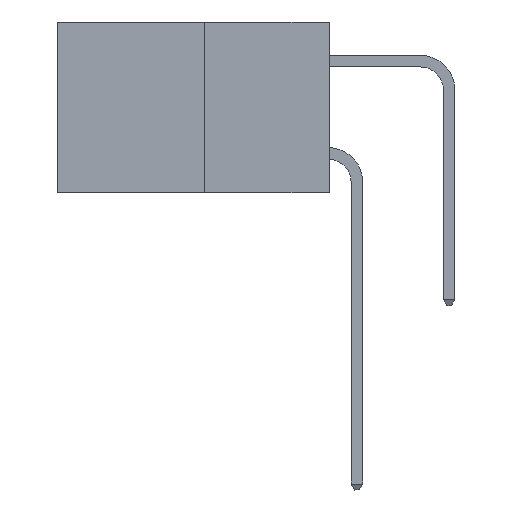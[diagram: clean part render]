
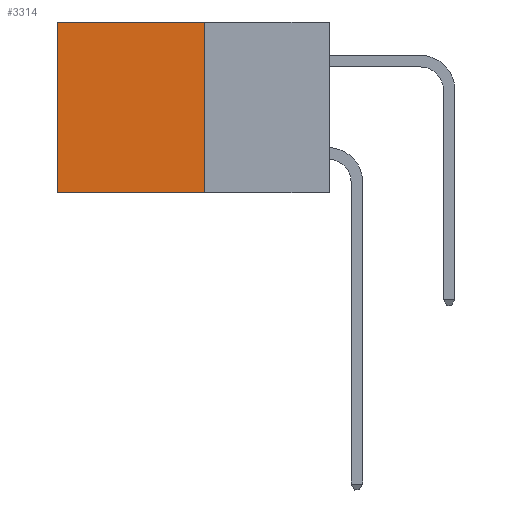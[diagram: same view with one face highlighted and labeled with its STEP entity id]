
A CAD part, left-side view. The second image highlights one B-rep face of the part: STEP entity #3314.
In plain terms, the highlighted planar face has unit normal (-1, 0, 0).
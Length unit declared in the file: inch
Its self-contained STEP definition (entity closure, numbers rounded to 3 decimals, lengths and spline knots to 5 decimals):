
#16 = AXIS2_PLACEMENT_3D ( 'NONE', #9712, #11095, #9691 ) ;
#469 = VECTOR ( 'NONE', #6134, 39.37008 ) ;
#1098 = VECTOR ( 'NONE', #6944, 39.37008 ) ;
#1236 = CARTESIAN_POINT ( 'NONE',  ( 0.277, 0.59, 0. ) ) ;
#1442 = CARTESIAN_POINT ( 'NONE',  ( 0.277, 0.27, -0.37 ) ) ;
#1795 = LINE ( 'NONE', #5856, #5884 ) ;
#3314 = ADVANCED_FACE ( 'NONE', ( #16702 ), #7497, .F. ) ;
#3338 = CARTESIAN_POINT ( 'NONE',  ( 0.277, 0.27, -0.37 ) ) ;
#3760 = CARTESIAN_POINT ( 'NONE',  ( 0.277, 0.59, -0.37 ) ) ;
#4749 = LINE ( 'NONE', #3760, #1098 ) ;
#5440 = EDGE_CURVE ( 'NONE', #11343, #13825, #4749, .T. ) ;
#5856 = CARTESIAN_POINT ( 'NONE',  ( 0.277, 0.27, 0. ) ) ;
#5884 = VECTOR ( 'NONE', #16940, 39.37008 ) ;
#6134 = DIRECTION ( 'NONE',  ( 0., 0., -1. ) ) ;
#6944 = DIRECTION ( 'NONE',  ( 0., 0., -1. ) ) ;
#7101 = VERTEX_POINT ( 'NONE', #13653 ) ;
#7150 = CARTESIAN_POINT ( 'NONE',  ( 0.277, 0.59, -0.37 ) ) ;
#7169 = EDGE_CURVE ( 'NONE', #7101, #11343, #1795, .T. ) ;
#7462 = VECTOR ( 'NONE', #9133, 39.37008 ) ;
#7497 = PLANE ( 'NONE',  #16 ) ;
#8184 = ORIENTED_EDGE ( 'NONE', *, *, #5440, .T. ) ;
#8253 = ORIENTED_EDGE ( 'NONE', *, *, #7169, .T. ) ;
#8892 = EDGE_CURVE ( 'NONE', #7101, #12126, #11355, .T. ) ;
#9133 = DIRECTION ( 'NONE',  ( 0., 1., 0. ) ) ;
#9691 = DIRECTION ( 'NONE',  ( 0., 0., -1. ) ) ;
#9712 = CARTESIAN_POINT ( 'NONE',  ( 0.277, 0.27, -0.37 ) ) ;
#11095 = DIRECTION ( 'NONE',  ( 1., 0., 0. ) ) ;
#11343 = VERTEX_POINT ( 'NONE', #1236 ) ;
#11355 = LINE ( 'NONE', #3338, #469 ) ;
#11489 = EDGE_LOOP ( 'NONE', ( #8184, #16342, #13719, #8253 ) ) ;
#11857 = EDGE_CURVE ( 'NONE', #12126, #13825, #14558, .T. ) ;
#12126 = VERTEX_POINT ( 'NONE', #1442 ) ;
#13653 = CARTESIAN_POINT ( 'NONE',  ( 0.277, 0.27, 0. ) ) ;
#13719 = ORIENTED_EDGE ( 'NONE', *, *, #8892, .F. ) ;
#13825 = VERTEX_POINT ( 'NONE', #7150 ) ;
#14558 = LINE ( 'NONE', #15729, #7462 ) ;
#15729 = CARTESIAN_POINT ( 'NONE',  ( 0.277, 0.27, -0.37 ) ) ;
#16342 = ORIENTED_EDGE ( 'NONE', *, *, #11857, .F. ) ;
#16702 = FACE_OUTER_BOUND ( 'NONE', #11489, .T. ) ;
#16940 = DIRECTION ( 'NONE',  ( 0., 1., 0. ) ) ;
